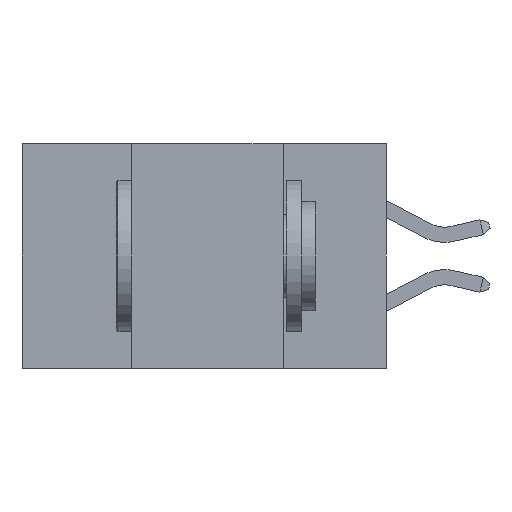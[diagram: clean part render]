
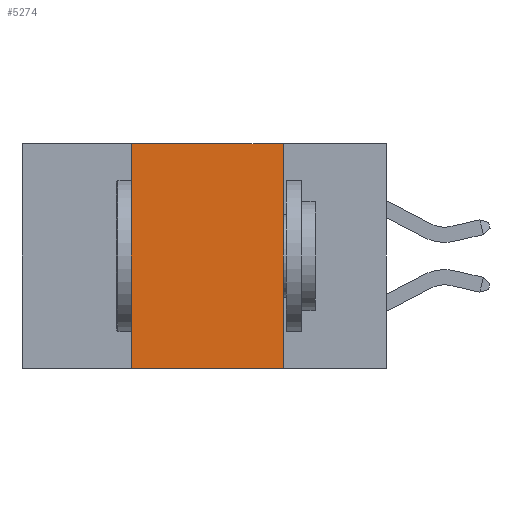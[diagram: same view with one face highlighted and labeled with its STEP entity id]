
A CAD part, left-side view. The second image highlights one B-rep face of the part: STEP entity #5274.
In plain terms, the highlighted planar face has unit normal (-1, 0, 0).
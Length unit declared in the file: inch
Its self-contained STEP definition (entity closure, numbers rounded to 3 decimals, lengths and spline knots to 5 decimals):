
#1002 = VECTOR ( 'NONE', #20487, 39.37008 ) ;
#2017 = EDGE_LOOP ( 'NONE', ( #26550, #9056, #4299, #16660 ) ) ;
#2037 = VECTOR ( 'NONE', #18929, 39.37008 ) ;
#3158 = VECTOR ( 'NONE', #27596, 39.37008 ) ;
#4210 = VERTEX_POINT ( 'NONE', #25251 ) ;
#4299 = ORIENTED_EDGE ( 'NONE', *, *, #26338, .F. ) ;
#4666 = FACE_OUTER_BOUND ( 'NONE', #2017, .T. ) ;
#5030 = CARTESIAN_POINT ( 'NONE',  ( 0., 0.6, -0.37 ) ) ;
#5274 = ADVANCED_FACE ( 'NONE', ( #4666 ), #9008, .F. ) ;
#6718 = CARTESIAN_POINT ( 'NONE',  ( 0., 0.6, 0. ) ) ;
#8982 = CARTESIAN_POINT ( 'NONE',  ( 0., 0.17, 0. ) ) ;
#9008 = PLANE ( 'NONE',  #19821 ) ;
#9056 = ORIENTED_EDGE ( 'NONE', *, *, #22054, .F. ) ;
#9589 = CARTESIAN_POINT ( 'NONE',  ( 0., 0.42, 0. ) ) ;
#14525 = LINE ( 'NONE', #27473, #25920 ) ;
#14565 = VERTEX_POINT ( 'NONE', #9589 ) ;
#16063 = CARTESIAN_POINT ( 'NONE',  ( 0., 0.17, -0.37 ) ) ;
#16288 = CARTESIAN_POINT ( 'NONE',  ( 0., 0.17, 0. ) ) ;
#16660 = ORIENTED_EDGE ( 'NONE', *, *, #29697, .T. ) ;
#18929 = DIRECTION ( 'NONE',  ( 0., -1., 0. ) ) ;
#19117 = LINE ( 'NONE', #5030, #2037 ) ;
#19821 = AXIS2_PLACEMENT_3D ( 'NONE', #6718, #22046, #29061 ) ;
#19942 = EDGE_CURVE ( 'NONE', #25161, #21970, #24827, .T. ) ;
#20487 = DIRECTION ( 'NONE',  ( 0., 0., -1. ) ) ;
#21970 = VERTEX_POINT ( 'NONE', #16063 ) ;
#22046 = DIRECTION ( 'NONE',  ( 1., 0., 0. ) ) ;
#22054 = EDGE_CURVE ( 'NONE', #14565, #25161, #26146, .T. ) ;
#24827 = LINE ( 'NONE', #8982, #1002 ) ;
#25161 = VERTEX_POINT ( 'NONE', #16288 ) ;
#25226 = DIRECTION ( 'NONE',  ( 0., 0., 1. ) ) ;
#25251 = CARTESIAN_POINT ( 'NONE',  ( 0., 0.42, -0.37 ) ) ;
#25377 = CARTESIAN_POINT ( 'NONE',  ( 0., 0.6, 0. ) ) ;
#25920 = VECTOR ( 'NONE', #25226, 39.37008 ) ;
#26146 = LINE ( 'NONE', #25377, #3158 ) ;
#26338 = EDGE_CURVE ( 'NONE', #4210, #14565, #14525, .T. ) ;
#26550 = ORIENTED_EDGE ( 'NONE', *, *, #19942, .F. ) ;
#27473 = CARTESIAN_POINT ( 'NONE',  ( 0., 0.42, 0. ) ) ;
#27596 = DIRECTION ( 'NONE',  ( 0., -1., 0. ) ) ;
#29061 = DIRECTION ( 'NONE',  ( 0., 0., -1. ) ) ;
#29697 = EDGE_CURVE ( 'NONE', #4210, #21970, #19117, .T. ) ;
